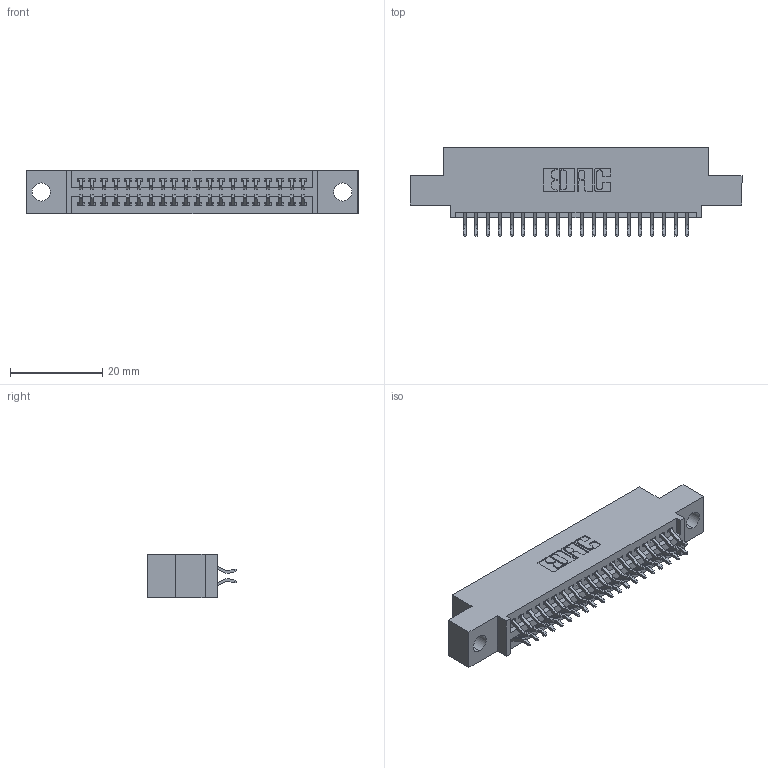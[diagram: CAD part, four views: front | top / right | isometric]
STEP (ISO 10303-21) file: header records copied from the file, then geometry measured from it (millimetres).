
FILE_DESCRIPTION (( 'STEP AP203' ), '1' );
FILE_NAME ('395-040-556-504.STEP', '2018-11-14T22:09:25', ( '' ), ( '' ), 'SwSTEP 2.0', 'SolidWorks 2016', '' );
FILE_SCHEMA (( 'CONFIG_CONTROL_DESIGN' ));
Length unit declared in the file: inch
Products named in the file (3): 395-040-556-504; 345-292-001_556 Tail; 345 Part_0.110 Offset - 0.156 Dia-TH
Assembly tree (41 placements, depth 2):
  395-040-556-504
    345 Part_0.110 Offset - 0.156 Dia-TH
    345-292-001_556 Tail  x40
Bounding box: 72.01 x 19.24 x 9.4 mm (x, y, z)
Volume: 6628 mm3; surface area: 9244.2 mm2
Topology: 41 solids, 41 shells, 2370 faces, 7033 edges, 4634 vertices
Faces by surface type: plane 1564, cylinder 806
Entity records: 19009 total; most frequent: CARTESIAN_POINT 3224, ORIENTED_EDGE 3146, DIRECTION 2857, EDGE_CURVE 1573, VECTOR 1353, LINE 1353, VERTEX_POINT 1046, AXIS2_PLACEMENT_3D 752
